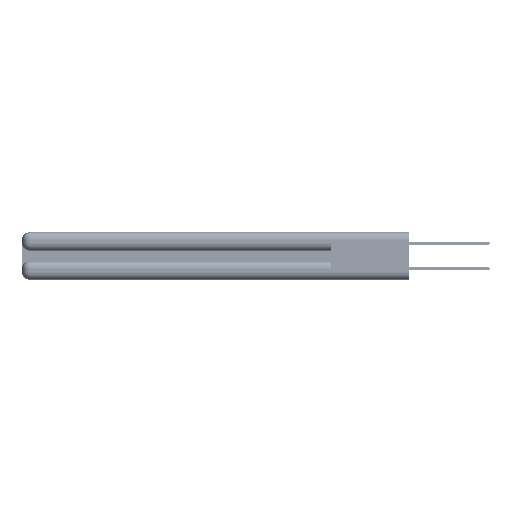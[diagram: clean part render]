
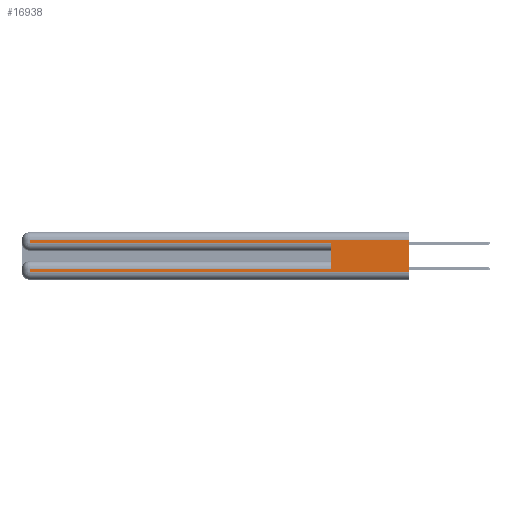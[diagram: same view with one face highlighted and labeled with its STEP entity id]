
A CAD part, left-side view. The second image highlights one B-rep face of the part: STEP entity #16938.
In plain terms, the highlighted planar face has unit normal (-1, 0, 0).
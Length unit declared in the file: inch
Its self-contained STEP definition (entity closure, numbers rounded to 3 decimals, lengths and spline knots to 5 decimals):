
#742 = EDGE_CURVE ( 'NONE', #12195, #5381, #32763, .T. ) ;
#1050 = EDGE_CURVE ( 'NONE', #47585, #12195, #21272, .T. ) ;
#1782 = EDGE_CURVE ( 'NONE', #50514, #20360, #50309, .T. ) ;
#3081 = DIRECTION ( 'NONE',  ( 0., 0., 1. ) ) ;
#5326 = LINE ( 'NONE', #49989, #17694 ) ;
#5381 = VERTEX_POINT ( 'NONE', #31557 ) ;
#6156 = CARTESIAN_POINT ( 'NONE',  ( 0., 2.94, 0.285 ) ) ;
#8208 = CARTESIAN_POINT ( 'NONE',  ( 0., 2.94, 0.37 ) ) ;
#9421 = DIRECTION ( 'NONE',  ( 0., 0., -1. ) ) ;
#11473 = VECTOR ( 'NONE', #45558, 39.37008 ) ;
#11788 = CARTESIAN_POINT ( 'NONE',  ( 0., 2.94, 0.31 ) ) ;
#12154 = CARTESIAN_POINT ( 'NONE',  ( 0., 0., 0.31 ) ) ;
#12195 = VERTEX_POINT ( 'NONE', #15295 ) ;
#12794 = ORIENTED_EDGE ( 'NONE', *, *, #1782, .T. ) ;
#13313 = VECTOR ( 'NONE', #25483, 39.37008 ) ;
#13456 = DIRECTION ( 'NONE',  ( 0., 1., 0. ) ) ;
#14817 = LINE ( 'NONE', #37700, #47863 ) ;
#15274 = CARTESIAN_POINT ( 'NONE',  ( 0., 0.6, 0.145 ) ) ;
#15295 = CARTESIAN_POINT ( 'NONE',  ( 0., 2.94, 0.06 ) ) ;
#15523 = DIRECTION ( 'NONE',  ( 0., 1., 0. ) ) ;
#16938 = ADVANCED_FACE ( 'NONE', ( #47459 ), #23082, .F. ) ;
#17694 = VECTOR ( 'NONE', #25568, 39.37008 ) ;
#18531 = ORIENTED_EDGE ( 'NONE', *, *, #742, .T. ) ;
#18792 = EDGE_CURVE ( 'NONE', #32044, #47585, #21432, .T. ) ;
#20360 = VERTEX_POINT ( 'NONE', #21062 ) ;
#20745 = CARTESIAN_POINT ( 'NONE',  ( 0., 0., 0.085 ) ) ;
#21062 = CARTESIAN_POINT ( 'NONE',  ( 0., 0.6, 0.285 ) ) ;
#21272 = LINE ( 'NONE', #8208, #11473 ) ;
#21432 = LINE ( 'NONE', #20745, #33673 ) ;
#21587 = ORIENTED_EDGE ( 'NONE', *, *, #49801, .T. ) ;
#23082 = PLANE ( 'NONE',  #41396 ) ;
#23276 = CARTESIAN_POINT ( 'NONE',  ( 0., 0.6, 0.085 ) ) ;
#23357 = DIRECTION ( 'NONE',  ( 0., -1., 0. ) ) ;
#24585 = CARTESIAN_POINT ( 'NONE',  ( 0., 0., 0.285 ) ) ;
#25483 = DIRECTION ( 'NONE',  ( 0., -1., 0. ) ) ;
#25568 = DIRECTION ( 'NONE',  ( 0., 0., -1. ) ) ;
#27224 = CARTESIAN_POINT ( 'NONE',  ( 0., 0., 0.37 ) ) ;
#27881 = VERTEX_POINT ( 'NONE', #11788 ) ;
#29214 = VECTOR ( 'NONE', #3081, 39.37008 ) ;
#31081 = LINE ( 'NONE', #15274, #29214 ) ;
#31557 = CARTESIAN_POINT ( 'NONE',  ( 0., 0., 0.06 ) ) ;
#31889 = EDGE_LOOP ( 'NONE', ( #47597, #21587, #42100, #12794, #46292, #34333, #35541, #18531 ) ) ;
#32044 = VERTEX_POINT ( 'NONE', #23276 ) ;
#32763 = LINE ( 'NONE', #39633, #35363 ) ;
#33673 = VECTOR ( 'NONE', #13456, 39.37008 ) ;
#34061 = DIRECTION ( 'NONE',  ( 0., 0., -1. ) ) ;
#34333 = ORIENTED_EDGE ( 'NONE', *, *, #18792, .T. ) ;
#34590 = CARTESIAN_POINT ( 'NONE',  ( 0., 0., 0.31 ) ) ;
#35363 = VECTOR ( 'NONE', #23357, 39.37008 ) ;
#35541 = ORIENTED_EDGE ( 'NONE', *, *, #1050, .T. ) ;
#37700 = CARTESIAN_POINT ( 'NONE',  ( 0., 2.94, 0.37 ) ) ;
#38191 = CARTESIAN_POINT ( 'NONE',  ( 0., 2.94, 0.085 ) ) ;
#39633 = CARTESIAN_POINT ( 'NONE',  ( 0., 0., 0.06 ) ) ;
#40833 = EDGE_CURVE ( 'NONE', #27881, #50514, #14817, .T. ) ;
#41396 = AXIS2_PLACEMENT_3D ( 'NONE', #27224, #52201, #34061 ) ;
#42100 = ORIENTED_EDGE ( 'NONE', *, *, #40833, .T. ) ;
#43971 = VERTEX_POINT ( 'NONE', #12154 ) ;
#45558 = DIRECTION ( 'NONE',  ( 0., 0., -1. ) ) ;
#45683 = EDGE_CURVE ( 'NONE', #32044, #20360, #31081, .T. ) ;
#45901 = VECTOR ( 'NONE', #15523, 39.37008 ) ;
#46292 = ORIENTED_EDGE ( 'NONE', *, *, #45683, .F. ) ;
#47426 = EDGE_CURVE ( 'NONE', #43971, #5381, #5326, .T. ) ;
#47459 = FACE_OUTER_BOUND ( 'NONE', #31889, .T. ) ;
#47585 = VERTEX_POINT ( 'NONE', #38191 ) ;
#47597 = ORIENTED_EDGE ( 'NONE', *, *, #47426, .F. ) ;
#47863 = VECTOR ( 'NONE', #9421, 39.37008 ) ;
#49801 = EDGE_CURVE ( 'NONE', #43971, #27881, #51110, .T. ) ;
#49989 = CARTESIAN_POINT ( 'NONE',  ( 0., 0., 0.37 ) ) ;
#50309 = LINE ( 'NONE', #24585, #13313 ) ;
#50514 = VERTEX_POINT ( 'NONE', #6156 ) ;
#51110 = LINE ( 'NONE', #34590, #45901 ) ;
#52201 = DIRECTION ( 'NONE',  ( 1., 0., 0. ) ) ;
